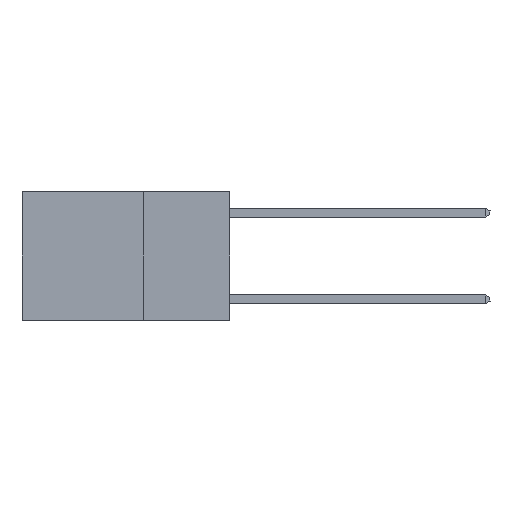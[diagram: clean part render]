
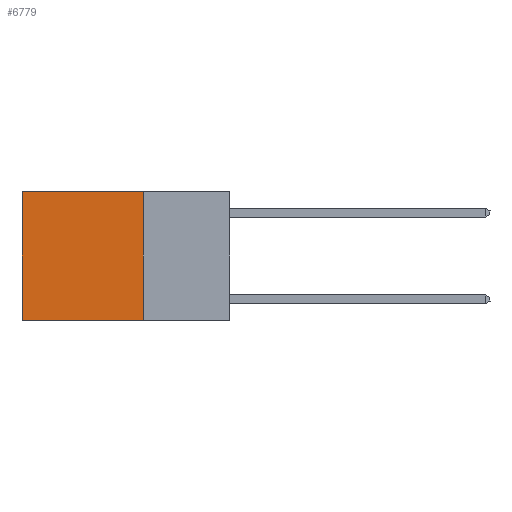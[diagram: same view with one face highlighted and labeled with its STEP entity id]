
A CAD part, left-side view. The second image highlights one B-rep face of the part: STEP entity #6779.
In plain terms, the highlighted planar face has unit normal (-1, 0, 0).
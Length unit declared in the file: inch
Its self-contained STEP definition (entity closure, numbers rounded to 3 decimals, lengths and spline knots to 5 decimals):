
#696 = LINE ( 'NONE', #10618, #12137 ) ;
#1298 = DIRECTION ( 'NONE',  ( 0., 0., -1. ) ) ;
#1322 = VECTOR ( 'NONE', #13898, 39.37008 ) ;
#1701 = VECTOR ( 'NONE', #3614, 39.37008 ) ;
#1749 = EDGE_CURVE ( 'NONE', #1760, #3922, #4655, .T. ) ;
#1760 = VERTEX_POINT ( 'NONE', #2592 ) ;
#1959 = DIRECTION ( 'NONE',  ( 0., 0., -1. ) ) ;
#2592 = CARTESIAN_POINT ( 'NONE',  ( 0.2625, 0.25, 0. ) ) ;
#3193 = CARTESIAN_POINT ( 'NONE',  ( 0.2625, 0.25, 0. ) ) ;
#3614 = DIRECTION ( 'NONE',  ( 0., 1., 0. ) ) ;
#3758 = CARTESIAN_POINT ( 'NONE',  ( 0.2625, 0.6, 0. ) ) ;
#3852 = EDGE_LOOP ( 'NONE', ( #10675, #9295, #12020, #7788 ) ) ;
#3922 = VERTEX_POINT ( 'NONE', #12208 ) ;
#4089 = VERTEX_POINT ( 'NONE', #6975 ) ;
#4655 = LINE ( 'NONE', #11373, #1701 ) ;
#5360 = AXIS2_PLACEMENT_3D ( 'NONE', #13988, #13912, #1959 ) ;
#6779 = ADVANCED_FACE ( 'NONE', ( #13115 ), #9710, .F. ) ;
#6975 = CARTESIAN_POINT ( 'NONE',  ( 0.2625, 0.25, -0.37 ) ) ;
#7190 = DIRECTION ( 'NONE',  ( 0., 1., 0. ) ) ;
#7485 = CARTESIAN_POINT ( 'NONE',  ( 0.2625, 0.6, -0.37 ) ) ;
#7788 = ORIENTED_EDGE ( 'NONE', *, *, #1749, .T. ) ;
#8226 = VECTOR ( 'NONE', #1298, 39.37008 ) ;
#8314 = LINE ( 'NONE', #3758, #1322 ) ;
#9295 = ORIENTED_EDGE ( 'NONE', *, *, #10972, .F. ) ;
#9301 = EDGE_CURVE ( 'NONE', #3922, #11073, #8314, .T. ) ;
#9710 = PLANE ( 'NONE',  #5360 ) ;
#10618 = CARTESIAN_POINT ( 'NONE',  ( 0.2625, 0.25, -0.37 ) ) ;
#10675 = ORIENTED_EDGE ( 'NONE', *, *, #9301, .T. ) ;
#10972 = EDGE_CURVE ( 'NONE', #4089, #11073, #696, .T. ) ;
#11073 = VERTEX_POINT ( 'NONE', #7485 ) ;
#11373 = CARTESIAN_POINT ( 'NONE',  ( 0.2625, 0.25, 0. ) ) ;
#12020 = ORIENTED_EDGE ( 'NONE', *, *, #13506, .F. ) ;
#12137 = VECTOR ( 'NONE', #7190, 39.37008 ) ;
#12156 = LINE ( 'NONE', #3193, #8226 ) ;
#12208 = CARTESIAN_POINT ( 'NONE',  ( 0.2625, 0.6, 0. ) ) ;
#13115 = FACE_OUTER_BOUND ( 'NONE', #3852, .T. ) ;
#13506 = EDGE_CURVE ( 'NONE', #1760, #4089, #12156, .T. ) ;
#13898 = DIRECTION ( 'NONE',  ( 0., 0., -1. ) ) ;
#13912 = DIRECTION ( 'NONE',  ( 1., 0., 0. ) ) ;
#13988 = CARTESIAN_POINT ( 'NONE',  ( 0.2625, 0.25, 0. ) ) ;
